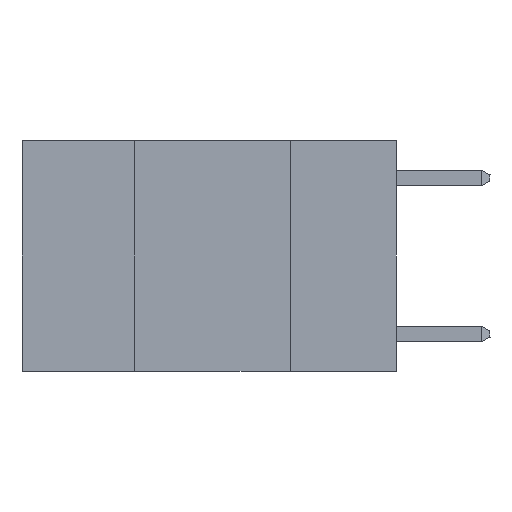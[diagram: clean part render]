
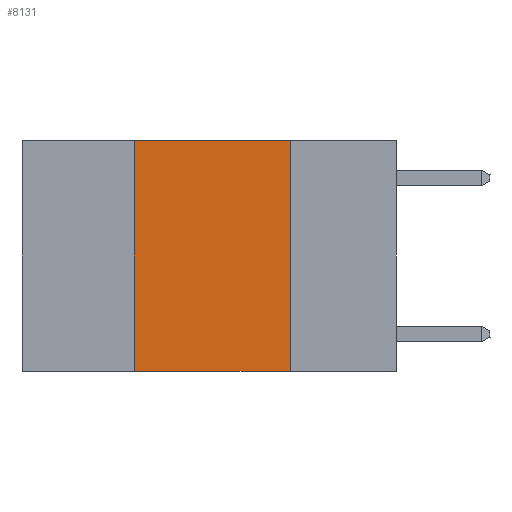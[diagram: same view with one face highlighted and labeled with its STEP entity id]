
A CAD part, left-side view. The second image highlights one B-rep face of the part: STEP entity #8131.
In plain terms, the highlighted planar face has unit normal (-1, 0, 0).
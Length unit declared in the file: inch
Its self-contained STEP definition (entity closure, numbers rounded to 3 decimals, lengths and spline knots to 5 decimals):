
#102 = VERTEX_POINT ( 'NONE', #12704 ) ;
#122 = VERTEX_POINT ( 'NONE', #4837 ) ;
#744 = ORIENTED_EDGE ( 'NONE', *, *, #10035, .T. ) ;
#853 = CARTESIAN_POINT ( 'NONE',  ( 0., 0.42, -0.37 ) ) ;
#1422 = DIRECTION ( 'NONE',  ( 0., 0., 1. ) ) ;
#1758 = CARTESIAN_POINT ( 'NONE',  ( 0., 0.42, 0. ) ) ;
#1841 = DIRECTION ( 'NONE',  ( 0., 0., -1. ) ) ;
#1879 = VECTOR ( 'NONE', #1422, 39.37008 ) ;
#1916 = FACE_OUTER_BOUND ( 'NONE', #8794, .T. ) ;
#2940 = CARTESIAN_POINT ( 'NONE',  ( 0., 0.6, 0. ) ) ;
#4302 = PLANE ( 'NONE',  #11612 ) ;
#4342 = CARTESIAN_POINT ( 'NONE',  ( 0., 0.17, -0.37 ) ) ;
#4837 = CARTESIAN_POINT ( 'NONE',  ( 0., 0.42, 0. ) ) ;
#5400 = VECTOR ( 'NONE', #5412, 39.37008 ) ;
#5412 = DIRECTION ( 'NONE',  ( 0., -1., 0. ) ) ;
#6086 = LINE ( 'NONE', #11868, #6829 ) ;
#6128 = VECTOR ( 'NONE', #12692, 39.37008 ) ;
#6373 = DIRECTION ( 'NONE',  ( 1., 0., 0. ) ) ;
#6744 = CARTESIAN_POINT ( 'NONE',  ( 0., 0.6, -0.37 ) ) ;
#6829 = VECTOR ( 'NONE', #11944, 39.37008 ) ;
#6886 = ORIENTED_EDGE ( 'NONE', *, *, #11075, .F. ) ;
#6971 = LINE ( 'NONE', #6744, #6128 ) ;
#7252 = VERTEX_POINT ( 'NONE', #853 ) ;
#8131 = ADVANCED_FACE ( 'NONE', ( #1916 ), #4302, .F. ) ;
#8559 = EDGE_CURVE ( 'NONE', #122, #102, #14630, .T. ) ;
#8794 = EDGE_LOOP ( 'NONE', ( #8905, #9756, #6886, #744 ) ) ;
#8905 = ORIENTED_EDGE ( 'NONE', *, *, #9225, .F. ) ;
#9225 = EDGE_CURVE ( 'NONE', #102, #10370, #6086, .T. ) ;
#9756 = ORIENTED_EDGE ( 'NONE', *, *, #8559, .F. ) ;
#10035 = EDGE_CURVE ( 'NONE', #7252, #10370, #6971, .T. ) ;
#10370 = VERTEX_POINT ( 'NONE', #4342 ) ;
#11075 = EDGE_CURVE ( 'NONE', #7252, #122, #14273, .T. ) ;
#11612 = AXIS2_PLACEMENT_3D ( 'NONE', #12081, #6373, #1841 ) ;
#11868 = CARTESIAN_POINT ( 'NONE',  ( 0., 0.17, 0. ) ) ;
#11944 = DIRECTION ( 'NONE',  ( 0., 0., -1. ) ) ;
#12081 = CARTESIAN_POINT ( 'NONE',  ( 0., 0.6, 0. ) ) ;
#12692 = DIRECTION ( 'NONE',  ( 0., -1., 0. ) ) ;
#12704 = CARTESIAN_POINT ( 'NONE',  ( 0., 0.17, 0. ) ) ;
#14273 = LINE ( 'NONE', #1758, #1879 ) ;
#14630 = LINE ( 'NONE', #2940, #5400 ) ;
